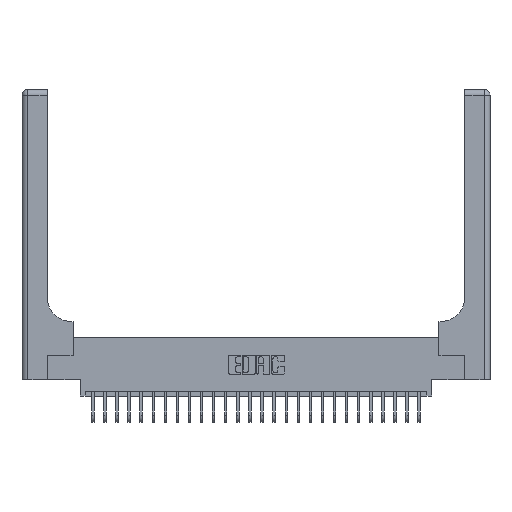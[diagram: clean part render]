
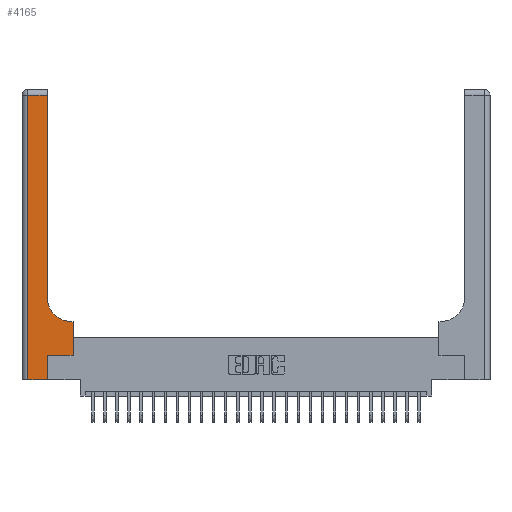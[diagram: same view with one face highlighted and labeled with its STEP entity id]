
A CAD part, top view. The second image highlights one B-rep face of the part: STEP entity #4165.
In plain terms, the highlighted planar face has unit normal (0, 0, 1).
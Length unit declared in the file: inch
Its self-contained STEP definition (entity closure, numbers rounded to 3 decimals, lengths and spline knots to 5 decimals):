
#47 = LINE ( 'NONE', #24154, #4711 ) ;
#451 = CARTESIAN_POINT ( 'NONE',  ( 0.26, 0.85, 0.37 ) ) ;
#573 = CARTESIAN_POINT ( 'NONE',  ( 0.06, 0., 0.37 ) ) ;
#599 = EDGE_CURVE ( 'NONE', #21300, #7551, #2033, .T. ) ;
#817 = EDGE_CURVE ( 'NONE', #4657, #11947, #20049, .T. ) ;
#1025 = ORIENTED_EDGE ( 'NONE', *, *, #26751, .T. ) ;
#1554 = DIRECTION ( 'NONE',  ( 1., 0., 0. ) ) ;
#1868 = CARTESIAN_POINT ( 'NONE',  ( 0.528, 0.25, 0.37 ) ) ;
#2033 = LINE ( 'NONE', #21236, #5632 ) ;
#2549 = CARTESIAN_POINT ( 'NONE',  ( 0., 0., 0.37 ) ) ;
#2565 = DIRECTION ( 'NONE',  ( 0., 1., 0. ) ) ;
#2727 = PLANE ( 'NONE',  #12884 ) ;
#2959 = DIRECTION ( 'NONE',  ( 0., -1., 0. ) ) ;
#3511 = VECTOR ( 'NONE', #6933, 39.37008 ) ;
#4165 = ADVANCED_FACE ( 'NONE', ( #13255 ), #2727, .F. ) ;
#4249 = CARTESIAN_POINT ( 'NONE',  ( 0.51, 0.85, 0.37 ) ) ;
#4657 = VERTEX_POINT ( 'NONE', #13027 ) ;
#4711 = VECTOR ( 'NONE', #25691, 39.37008 ) ;
#5259 = ORIENTED_EDGE ( 'NONE', *, *, #6427, .T. ) ;
#5590 = VERTEX_POINT ( 'NONE', #451 ) ;
#5632 = VECTOR ( 'NONE', #10601, 39.37008 ) ;
#6253 = VECTOR ( 'NONE', #2959, 39.37008 ) ;
#6427 = EDGE_CURVE ( 'NONE', #11947, #25204, #23761, .T. ) ;
#6704 = LINE ( 'NONE', #15245, #13021 ) ;
#6933 = DIRECTION ( 'NONE',  ( 1., 0., 0. ) ) ;
#6967 = DIRECTION ( 'NONE',  ( -1., 0., 0. ) ) ;
#7317 = CARTESIAN_POINT ( 'NONE',  ( 0.26, 2.94, 0.37 ) ) ;
#7370 = DIRECTION ( 'NONE',  ( 0., 0., -1. ) ) ;
#7551 = VERTEX_POINT ( 'NONE', #26583 ) ;
#8972 = LINE ( 'NONE', #20145, #16575 ) ;
#10601 = DIRECTION ( 'NONE',  ( -1., 0., 0. ) ) ;
#11388 = VERTEX_POINT ( 'NONE', #13599 ) ;
#11701 = CARTESIAN_POINT ( 'NONE',  ( 0.265, 0., 0.37 ) ) ;
#11947 = VERTEX_POINT ( 'NONE', #1868 ) ;
#12033 = EDGE_CURVE ( 'NONE', #5590, #21300, #47, .T. ) ;
#12127 = ORIENTED_EDGE ( 'NONE', *, *, #599, .T. ) ;
#12884 = AXIS2_PLACEMENT_3D ( 'NONE', #21801, #7370, #6967 ) ;
#12932 = CARTESIAN_POINT ( 'NONE',  ( 0.06, 3., 0.37 ) ) ;
#13021 = VECTOR ( 'NONE', #17741, 39.37008 ) ;
#13027 = CARTESIAN_POINT ( 'NONE',  ( 0.265, 0.25, 0.37 ) ) ;
#13059 = VERTEX_POINT ( 'NONE', #11701 ) ;
#13255 = FACE_OUTER_BOUND ( 'NONE', #25435, .T. ) ;
#13599 = CARTESIAN_POINT ( 'NONE',  ( 0.51, 0.6, 0.37 ) ) ;
#13980 = ORIENTED_EDGE ( 'NONE', *, *, #18783, .T. ) ;
#14513 = VERTEX_POINT ( 'NONE', #573 ) ;
#15031 = LINE ( 'NONE', #12932, #6253 ) ;
#15245 = CARTESIAN_POINT ( 'NONE',  ( 0.26, 0.6, 0.37 ) ) ;
#16298 = DIRECTION ( 'NONE',  ( 1., 0., 0. ) ) ;
#16575 = VECTOR ( 'NONE', #24229, 39.37008 ) ;
#16591 = EDGE_CURVE ( 'NONE', #11388, #5590, #17399, .T. ) ;
#17393 = CARTESIAN_POINT ( 'NONE',  ( 0.528, 0.6, 0.37 ) ) ;
#17399 = CIRCLE ( 'NONE', #21881, 0.25 ) ;
#17741 = DIRECTION ( 'NONE',  ( -1., 0., 0. ) ) ;
#17820 = CARTESIAN_POINT ( 'NONE',  ( 0.265, 0.25, 0.37 ) ) ;
#18589 = ORIENTED_EDGE ( 'NONE', *, *, #22958, .T. ) ;
#18668 = DIRECTION ( 'NONE',  ( 0., 0., -1. ) ) ;
#18728 = ORIENTED_EDGE ( 'NONE', *, *, #16591, .T. ) ;
#18783 = EDGE_CURVE ( 'NONE', #14513, #13059, #25963, .T. ) ;
#20049 = LINE ( 'NONE', #17820, #24794 ) ;
#20145 = CARTESIAN_POINT ( 'NONE',  ( 0.265, 0., 0.37 ) ) ;
#21233 = ORIENTED_EDGE ( 'NONE', *, *, #817, .T. ) ;
#21236 = CARTESIAN_POINT ( 'NONE',  ( 0., 2.94, 0.37 ) ) ;
#21300 = VERTEX_POINT ( 'NONE', #7317 ) ;
#21639 = CARTESIAN_POINT ( 'NONE',  ( 0.528, 0.25, 0.37 ) ) ;
#21801 = CARTESIAN_POINT ( 'NONE',  ( 0., 3., 0.37 ) ) ;
#21881 = AXIS2_PLACEMENT_3D ( 'NONE', #4249, #18668, #1554 ) ;
#22958 = EDGE_CURVE ( 'NONE', #25204, #11388, #6704, .T. ) ;
#23761 = LINE ( 'NONE', #21639, #25228 ) ;
#23944 = ORIENTED_EDGE ( 'NONE', *, *, #26174, .T. ) ;
#24154 = CARTESIAN_POINT ( 'NONE',  ( 0.26, 3., 0.37 ) ) ;
#24229 = DIRECTION ( 'NONE',  ( 0., 1., 0. ) ) ;
#24794 = VECTOR ( 'NONE', #16298, 39.37008 ) ;
#25204 = VERTEX_POINT ( 'NONE', #17393 ) ;
#25228 = VECTOR ( 'NONE', #2565, 39.37008 ) ;
#25435 = EDGE_LOOP ( 'NONE', ( #25812, #12127, #23944, #13980, #1025, #21233, #5259, #18589, #18728 ) ) ;
#25691 = DIRECTION ( 'NONE',  ( 0., 1., 0. ) ) ;
#25812 = ORIENTED_EDGE ( 'NONE', *, *, #12033, .T. ) ;
#25963 = LINE ( 'NONE', #2549, #3511 ) ;
#26174 = EDGE_CURVE ( 'NONE', #7551, #14513, #15031, .T. ) ;
#26583 = CARTESIAN_POINT ( 'NONE',  ( 0.06, 2.94, 0.37 ) ) ;
#26751 = EDGE_CURVE ( 'NONE', #13059, #4657, #8972, .T. ) ;
